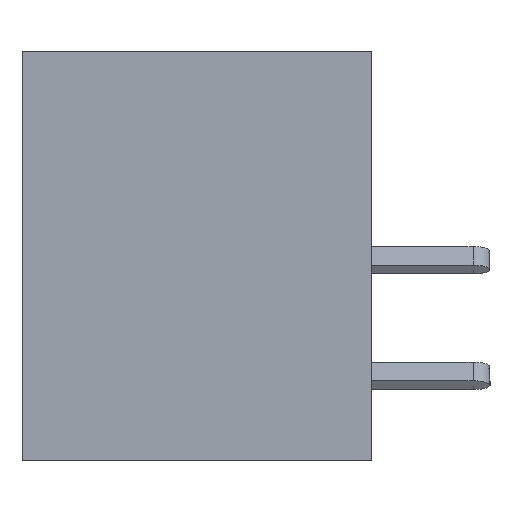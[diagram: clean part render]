
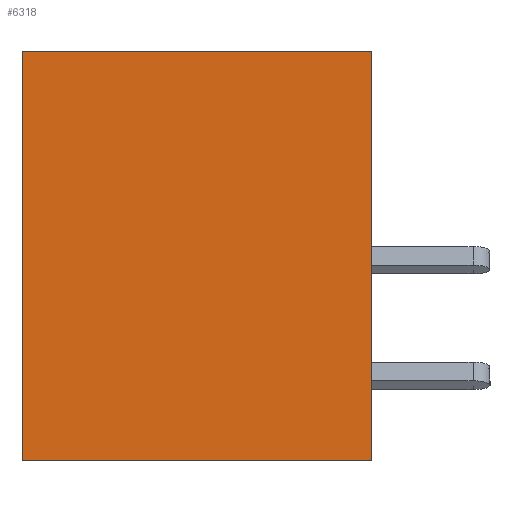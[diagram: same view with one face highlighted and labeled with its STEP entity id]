
A CAD part, left-side view. The second image highlights one B-rep face of the part: STEP entity #6318.
In plain terms, the highlighted planar face has unit normal (-1, 0, 0).
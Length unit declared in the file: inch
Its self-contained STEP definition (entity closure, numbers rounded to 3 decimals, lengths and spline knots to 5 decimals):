
#66 = LINE ( 'NONE', #27264, #15673 ) ;
#1558 = ORIENTED_EDGE ( 'NONE', *, *, #3372, .F. ) ;
#3372 = EDGE_CURVE ( 'NONE', #25702, #23885, #18135, .T. ) ;
#3766 = FACE_OUTER_BOUND ( 'NONE', #28464, .T. ) ;
#4273 = CARTESIAN_POINT ( 'NONE',  ( 0., 0.453, -0.531 ) ) ;
#4721 = EDGE_CURVE ( 'NONE', #6440, #12060, #66, .T. ) ;
#5034 = ORIENTED_EDGE ( 'NONE', *, *, #10707, .F. ) ;
#6318 = ADVANCED_FACE ( 'NONE', ( #3766 ), #22994, .F. ) ;
#6440 = VERTEX_POINT ( 'NONE', #4273 ) ;
#6459 = DIRECTION ( 'NONE',  ( 0., -1., 0. ) ) ;
#7314 = DIRECTION ( 'NONE',  ( 0., -1., 0. ) ) ;
#9112 = CARTESIAN_POINT ( 'NONE',  ( 0., 0.453, 0. ) ) ;
#9168 = CARTESIAN_POINT ( 'NONE',  ( 0., 0.453, 0. ) ) ;
#9940 = AXIS2_PLACEMENT_3D ( 'NONE', #16363, #25285, #19246 ) ;
#10707 = EDGE_CURVE ( 'NONE', #6440, #25702, #24325, .T. ) ;
#10837 = CARTESIAN_POINT ( 'NONE',  ( 0., 0.453, 0. ) ) ;
#11795 = VECTOR ( 'NONE', #21359, 39.37008 ) ;
#12060 = VERTEX_POINT ( 'NONE', #23362 ) ;
#13948 = VECTOR ( 'NONE', #19851, 39.37008 ) ;
#14426 = CARTESIAN_POINT ( 'NONE',  ( 0., 0., 0. ) ) ;
#15673 = VECTOR ( 'NONE', #7314, 39.37008 ) ;
#16363 = CARTESIAN_POINT ( 'NONE',  ( 0., 0.453, 0. ) ) ;
#16438 = ORIENTED_EDGE ( 'NONE', *, *, #20010, .T. ) ;
#17674 = CARTESIAN_POINT ( 'NONE',  ( 0., 0., 0. ) ) ;
#18135 = LINE ( 'NONE', #10837, #25435 ) ;
#19246 = DIRECTION ( 'NONE',  ( 0., 0., -1. ) ) ;
#19851 = DIRECTION ( 'NONE',  ( 0., 0., 1. ) ) ;
#20010 = EDGE_CURVE ( 'NONE', #12060, #23885, #26691, .T. ) ;
#21359 = DIRECTION ( 'NONE',  ( 0., 0., 1. ) ) ;
#22994 = PLANE ( 'NONE',  #9940 ) ;
#23362 = CARTESIAN_POINT ( 'NONE',  ( 0., 0., -0.531 ) ) ;
#23885 = VERTEX_POINT ( 'NONE', #17674 ) ;
#24325 = LINE ( 'NONE', #9168, #13948 ) ;
#24351 = ORIENTED_EDGE ( 'NONE', *, *, #4721, .T. ) ;
#25285 = DIRECTION ( 'NONE',  ( 1., 0., 0. ) ) ;
#25435 = VECTOR ( 'NONE', #6459, 39.37008 ) ;
#25702 = VERTEX_POINT ( 'NONE', #9112 ) ;
#26691 = LINE ( 'NONE', #14426, #11795 ) ;
#27264 = CARTESIAN_POINT ( 'NONE',  ( 0., 0.453, -0.531 ) ) ;
#28464 = EDGE_LOOP ( 'NONE', ( #16438, #1558, #5034, #24351 ) ) ;
